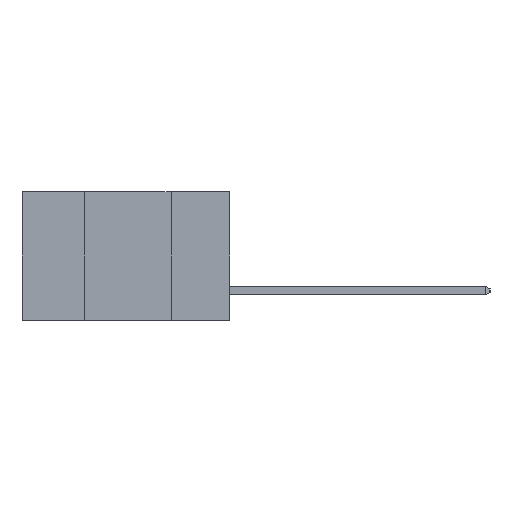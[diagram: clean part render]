
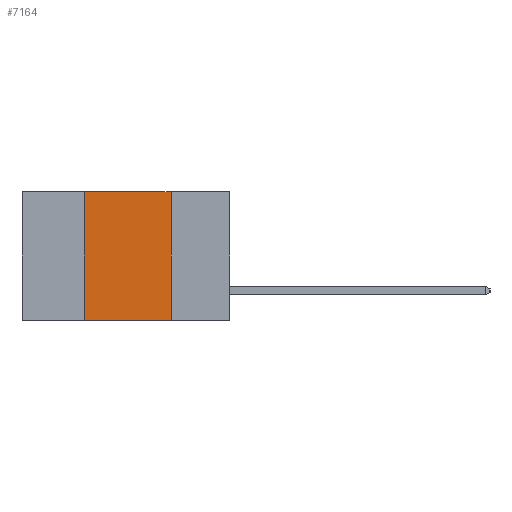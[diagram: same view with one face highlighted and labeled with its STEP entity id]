
A CAD part, left-side view. The second image highlights one B-rep face of the part: STEP entity #7164.
In plain terms, the highlighted planar face has unit normal (-1, 0, 0).
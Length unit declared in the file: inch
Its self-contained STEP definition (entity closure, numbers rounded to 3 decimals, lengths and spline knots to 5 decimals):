
#323 = CARTESIAN_POINT ( 'NONE',  ( 0., 0.6, -0.37 ) ) ;
#1025 = VERTEX_POINT ( 'NONE', #15959 ) ;
#1223 = LINE ( 'NONE', #1844, #6504 ) ;
#1792 = DIRECTION ( 'NONE',  ( 0., 0., -1. ) ) ;
#1844 = CARTESIAN_POINT ( 'NONE',  ( 0., 0.17, 0. ) ) ;
#1994 = ORIENTED_EDGE ( 'NONE', *, *, #8351, .F. ) ;
#2540 = EDGE_CURVE ( 'NONE', #24597, #4389, #9510, .T. ) ;
#2937 = DIRECTION ( 'NONE',  ( 0., 0., 1. ) ) ;
#4086 = CARTESIAN_POINT ( 'NONE',  ( 0., 0.17, -0.37 ) ) ;
#4389 = VERTEX_POINT ( 'NONE', #4086 ) ;
#4565 = VECTOR ( 'NONE', #21013, 39.37008 ) ;
#5637 = DIRECTION ( 'NONE',  ( 0., 0., -1. ) ) ;
#5699 = DIRECTION ( 'NONE',  ( 1., 0., 0. ) ) ;
#5732 = PLANE ( 'NONE',  #6725 ) ;
#6078 = CARTESIAN_POINT ( 'NONE',  ( 0., 0.6, 0. ) ) ;
#6504 = VECTOR ( 'NONE', #1792, 39.37008 ) ;
#6725 = AXIS2_PLACEMENT_3D ( 'NONE', #6078, #5699, #5637 ) ;
#7164 = ADVANCED_FACE ( 'NONE', ( #11442 ), #5732, .F. ) ;
#7376 = EDGE_CURVE ( 'NONE', #1025, #4389, #1223, .T. ) ;
#8351 = EDGE_CURVE ( 'NONE', #22899, #1025, #9193, .T. ) ;
#8498 = ORIENTED_EDGE ( 'NONE', *, *, #15756, .F. ) ;
#9193 = LINE ( 'NONE', #13328, #4565 ) ;
#9510 = LINE ( 'NONE', #323, #24370 ) ;
#11328 = VECTOR ( 'NONE', #2937, 39.37008 ) ;
#11442 = FACE_OUTER_BOUND ( 'NONE', #14576, .T. ) ;
#12791 = CARTESIAN_POINT ( 'NONE',  ( 0., 0.42, 0. ) ) ;
#13328 = CARTESIAN_POINT ( 'NONE',  ( 0., 0.6, 0. ) ) ;
#14052 = ORIENTED_EDGE ( 'NONE', *, *, #7376, .F. ) ;
#14576 = EDGE_LOOP ( 'NONE', ( #14052, #1994, #8498, #25138 ) ) ;
#15756 = EDGE_CURVE ( 'NONE', #24597, #22899, #16544, .T. ) ;
#15959 = CARTESIAN_POINT ( 'NONE',  ( 0., 0.17, 0. ) ) ;
#16544 = LINE ( 'NONE', #12791, #11328 ) ;
#18833 = CARTESIAN_POINT ( 'NONE',  ( 0., 0.42, -0.37 ) ) ;
#21013 = DIRECTION ( 'NONE',  ( 0., -1., 0. ) ) ;
#21228 = DIRECTION ( 'NONE',  ( 0., -1., 0. ) ) ;
#22899 = VERTEX_POINT ( 'NONE', #23009 ) ;
#23009 = CARTESIAN_POINT ( 'NONE',  ( 0., 0.42, 0. ) ) ;
#24370 = VECTOR ( 'NONE', #21228, 39.37008 ) ;
#24597 = VERTEX_POINT ( 'NONE', #18833 ) ;
#25138 = ORIENTED_EDGE ( 'NONE', *, *, #2540, .T. ) ;
